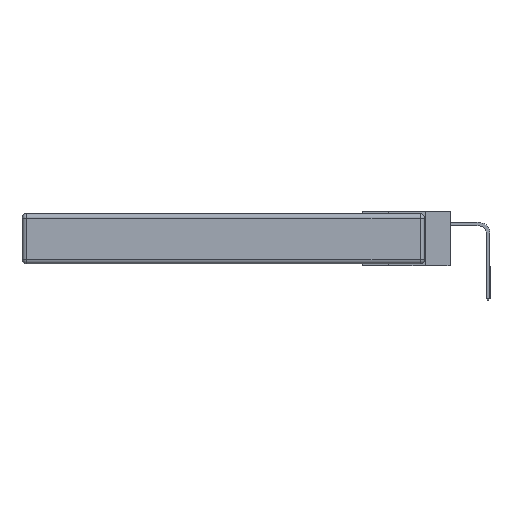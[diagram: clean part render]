
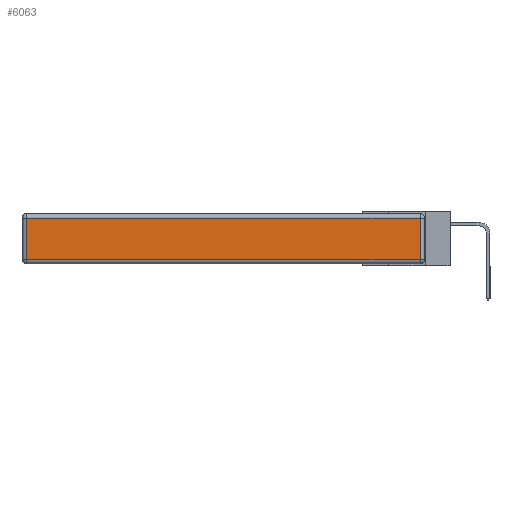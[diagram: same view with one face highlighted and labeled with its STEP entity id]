
A CAD part, left-side view. The second image highlights one B-rep face of the part: STEP entity #6063.
In plain terms, the highlighted planar face has unit normal (-1, 0, 0).
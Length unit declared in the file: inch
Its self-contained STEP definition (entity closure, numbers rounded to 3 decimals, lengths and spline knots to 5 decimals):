
#210 = CARTESIAN_POINT ( 'NONE',  ( 0., 2.75, -0.03 ) ) ;
#352 = LINE ( 'NONE', #858, #6370 ) ;
#429 = VERTEX_POINT ( 'NONE', #8539 ) ;
#453 = AXIS2_PLACEMENT_3D ( 'NONE', #6409, #8261, #2701 ) ;
#858 = CARTESIAN_POINT ( 'NONE',  ( 0., 0., -0.313 ) ) ;
#1348 = EDGE_CURVE ( 'NONE', #2198, #429, #7658, .T. ) ;
#1352 = ORIENTED_EDGE ( 'NONE', *, *, #1348, .T. ) ;
#1692 = ORIENTED_EDGE ( 'NONE', *, *, #5785, .T. ) ;
#2186 = DIRECTION ( 'NONE',  ( 0., -1., 0. ) ) ;
#2198 = VERTEX_POINT ( 'NONE', #7920 ) ;
#2701 = DIRECTION ( 'NONE',  ( 0., 0., 1. ) ) ;
#3329 = VECTOR ( 'NONE', #8167, 39.37008 ) ;
#4123 = VECTOR ( 'NONE', #10900, 39.37008 ) ;
#4195 = ORIENTED_EDGE ( 'NONE', *, *, #7952, .T. ) ;
#4589 = EDGE_CURVE ( 'NONE', #429, #5678, #352, .T. ) ;
#4813 = VERTEX_POINT ( 'NONE', #5198 ) ;
#5198 = CARTESIAN_POINT ( 'NONE',  ( 0., 0.03, -0.03 ) ) ;
#5462 = CARTESIAN_POINT ( 'NONE',  ( 0., 2.72, -0.343 ) ) ;
#5482 = ORIENTED_EDGE ( 'NONE', *, *, #4589, .T. ) ;
#5678 = VERTEX_POINT ( 'NONE', #7510 ) ;
#5745 = FACE_OUTER_BOUND ( 'NONE', #6965, .T. ) ;
#5785 = EDGE_CURVE ( 'NONE', #4813, #2198, #11865, .T. ) ;
#5893 = VECTOR ( 'NONE', #9215, 39.37008 ) ;
#6063 = ADVANCED_FACE ( 'NONE', ( #5745 ), #11053, .T. ) ;
#6370 = VECTOR ( 'NONE', #2186, 39.37008 ) ;
#6409 = CARTESIAN_POINT ( 'NONE',  ( 0., 0., -0.343 ) ) ;
#6965 = EDGE_LOOP ( 'NONE', ( #5482, #4195, #1692, #1352 ) ) ;
#7510 = CARTESIAN_POINT ( 'NONE',  ( 0., 0.03, -0.313 ) ) ;
#7658 = LINE ( 'NONE', #5462, #5893 ) ;
#7920 = CARTESIAN_POINT ( 'NONE',  ( 0., 2.72, -0.03 ) ) ;
#7952 = EDGE_CURVE ( 'NONE', #5678, #4813, #8292, .T. ) ;
#8167 = DIRECTION ( 'NONE',  ( 0., 0., 1. ) ) ;
#8261 = DIRECTION ( 'NONE',  ( -1., 0., 0. ) ) ;
#8292 = LINE ( 'NONE', #9075, #3329 ) ;
#8539 = CARTESIAN_POINT ( 'NONE',  ( 0., 2.72, -0.313 ) ) ;
#9075 = CARTESIAN_POINT ( 'NONE',  ( 0., 0.03, -0.343 ) ) ;
#9215 = DIRECTION ( 'NONE',  ( 0., 0., -1. ) ) ;
#10900 = DIRECTION ( 'NONE',  ( 0., 1., 0. ) ) ;
#11053 = PLANE ( 'NONE',  #453 ) ;
#11865 = LINE ( 'NONE', #210, #4123 ) ;
